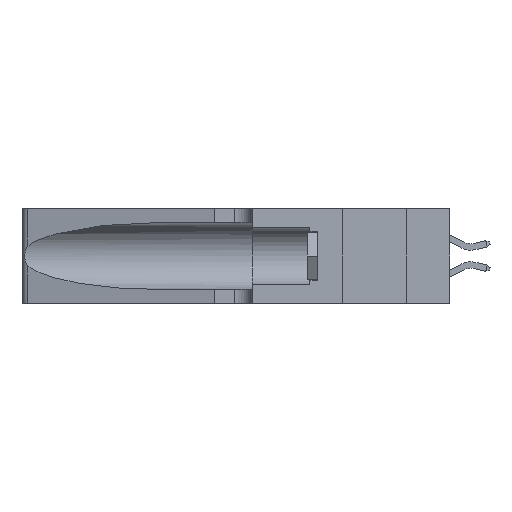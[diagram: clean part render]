
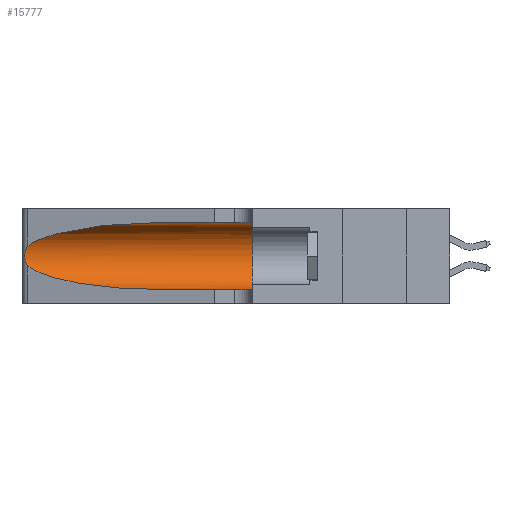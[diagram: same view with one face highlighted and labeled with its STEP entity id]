
A CAD part, left-side view. The second image highlights one B-rep face of the part: STEP entity #15777.
In plain terms, the highlighted cylindrical face has radius 3.308 mm (diameter 6.617 mm), a partial arc.
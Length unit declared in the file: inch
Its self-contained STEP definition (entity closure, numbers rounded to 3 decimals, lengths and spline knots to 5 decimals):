
#807 = DIRECTION ( 'NONE',  ( 0., -1., 0. ) ) ;
#808 = AXIS2_PLACEMENT_3D ( 'NONE', #12505, #12678, #12764 ) ;
#862 = CARTESIAN_POINT ( 'NONE',  ( 0.18966, 0.96281, 0.05475 ) ) ;
#995 = EDGE_CURVE ( 'NONE', #19436, #9835, #7386, .T. ) ;
#1857 = CARTESIAN_POINT ( 'NONE',  ( 0.25854, 1.2359, 0.20912 ) ) ;
#1946 = CARTESIAN_POINT ( 'NONE',  ( 0.26075, 1.23896, 0.178 ) ) ;
#2101 = CARTESIAN_POINT ( 'NONE',  ( 0.26017, 1.23833, 0.17102 ) ) ;
#2429 = VECTOR ( 'NONE', #807, 39.37008 ) ;
#4340 = CARTESIAN_POINT ( 'NONE',  ( 0.1305, 0.72297, 0.05475 ) ) ;
#4349 = CARTESIAN_POINT ( 'NONE',  ( 0.1305, 0.35, 0.31525 ) ) ;
#5874 = CARTESIAN_POINT ( 'NONE',  ( 0.1305, 1.61858, 0.31525 ) ) ;
#6465 = EDGE_LOOP ( 'NONE', ( #8279, #24829, #11909, #16820, #25106, #7461 ) ) ;
#6874 = EDGE_CURVE ( 'NONE', #16310, #11037, #12631, .T. ) ;
#6916 =( BOUNDED_CURVE ( )  B_SPLINE_CURVE ( 3, ( #19974, #18110, #862, #18564 ),
 .UNSPECIFIED., .F., .T. ) 
 B_SPLINE_CURVE_WITH_KNOTS ( ( 4, 4 ),
 ( 3.44316, 4.71239 ),
 .UNSPECIFIED. ) 
 CURVE ( )  GEOMETRIC_REPRESENTATION_ITEM ( )  RATIONAL_B_SPLINE_CURVE ( ( 1., 0.87, 0.87, 1. ) ) 
 REPRESENTATION_ITEM ( '' )  );
#7386 = B_SPLINE_CURVE_WITH_KNOTS ( 'NONE', 3,
 ( #21714, #17870, #23707, #9993, #1857, #23624, #19993, #1946, #2101, #13982, #15690, #25715, #15786, #7904 ),
 .UNSPECIFIED., .F., .F.,
 ( 4, 2, 2, 2, 2, 2, 4 ),
 ( 0., 0.00027, 0.00053, 0.00107, 0.0016, 0.00187, 0.00214 ),
 .UNSPECIFIED. ) ;
#7461 = ORIENTED_EDGE ( 'NONE', *, *, #15427, .F. ) ;
#7904 = CARTESIAN_POINT ( 'NONE',  ( 0.25487, 1.22718, 0.14631 ) ) ;
#8279 = ORIENTED_EDGE ( 'NONE', *, *, #11828, .T. ) ;
#8704 = DIRECTION ( 'NONE',  ( 0., 0., 1. ) ) ;
#9835 = VERTEX_POINT ( 'NONE', #12852 ) ;
#9993 = CARTESIAN_POINT ( 'NONE',  ( 0.25787, 1.23484, 0.2124 ) ) ;
#10057 = CARTESIAN_POINT ( 'NONE',  ( 0.25487, 1.22718, 0.22369 ) ) ;
#10873 =( BOUNDED_CURVE ( )  B_SPLINE_CURVE ( 3, ( #22787, #15052, #18729, #24969 ),
 .UNSPECIFIED., .F., .F. ) 
 B_SPLINE_CURVE_WITH_KNOTS ( ( 4, 4 ),
 ( 1.5708, 2.84003 ),
 .UNSPECIFIED. ) 
 CURVE ( )  GEOMETRIC_REPRESENTATION_ITEM ( )  RATIONAL_B_SPLINE_CURVE ( ( 1., 0.87, 0.87, 1. ) ) 
 REPRESENTATION_ITEM ( '' )  );
#11037 = VERTEX_POINT ( 'NONE', #16438 ) ;
#11586 = CYLINDRICAL_SURFACE ( 'NONE', #808, 0.13025 ) ;
#11828 = EDGE_CURVE ( 'NONE', #23755, #19436, #10873, .T. ) ;
#11909 = ORIENTED_EDGE ( 'NONE', *, *, #12552, .T. ) ;
#12505 = CARTESIAN_POINT ( 'NONE',  ( 0.1305, 1.61858, 0.185 ) ) ;
#12552 = EDGE_CURVE ( 'NONE', #9835, #16310, #6916, .T. ) ;
#12631 = LINE ( 'NONE', #16578, #2429 ) ;
#12678 = DIRECTION ( 'NONE',  ( 0., -1., 0. ) ) ;
#12764 = DIRECTION ( 'NONE',  ( 0., 0., -1. ) ) ;
#12852 = CARTESIAN_POINT ( 'NONE',  ( 0.25487, 1.22718, 0.14631 ) ) ;
#13520 = DIRECTION ( 'NONE',  ( 0., -1., 0. ) ) ;
#13982 = CARTESIAN_POINT ( 'NONE',  ( 0.25856, 1.23593, 0.16098 ) ) ;
#15052 = CARTESIAN_POINT ( 'NONE',  ( 0.18966, 0.96281, 0.31525 ) ) ;
#15427 = EDGE_CURVE ( 'NONE', #23755, #18239, #17205, .T. ) ;
#15690 = CARTESIAN_POINT ( 'NONE',  ( 0.25789, 1.23486, 0.15765 ) ) ;
#15777 = ADVANCED_FACE ( 'NONE', ( #24671 ), #11586, .F. ) ;
#15786 = CARTESIAN_POINT ( 'NONE',  ( 0.25555, 1.22993, 0.14849 ) ) ;
#16310 = VERTEX_POINT ( 'NONE', #4340 ) ;
#16438 = CARTESIAN_POINT ( 'NONE',  ( 0.1305, 0.35, 0.05475 ) ) ;
#16578 = CARTESIAN_POINT ( 'NONE',  ( 0.1305, 1.61858, 0.05475 ) ) ;
#16820 = ORIENTED_EDGE ( 'NONE', *, *, #6874, .T. ) ;
#17205 = LINE ( 'NONE', #5874, #19716 ) ;
#17869 = EDGE_CURVE ( 'NONE', #18239, #11037, #23369, .T. ) ;
#17870 = CARTESIAN_POINT ( 'NONE',  ( 0.25555, 1.22994, 0.2215 ) ) ;
#18110 = CARTESIAN_POINT ( 'NONE',  ( 0.2373, 1.15595, 0.08982 ) ) ;
#18239 = VERTEX_POINT ( 'NONE', #4349 ) ;
#18487 = CARTESIAN_POINT ( 'NONE',  ( 0.1305, 0.35, 0.185 ) ) ;
#18564 = CARTESIAN_POINT ( 'NONE',  ( 0.1305, 0.72297, 0.05475 ) ) ;
#18679 = DIRECTION ( 'NONE',  ( 0., 1., 0. ) ) ;
#18729 = CARTESIAN_POINT ( 'NONE',  ( 0.2373, 1.15595, 0.28018 ) ) ;
#19436 = VERTEX_POINT ( 'NONE', #10057 ) ;
#19716 = VECTOR ( 'NONE', #13520, 39.37008 ) ;
#19974 = CARTESIAN_POINT ( 'NONE',  ( 0.25487, 1.22718, 0.14631 ) ) ;
#19993 = CARTESIAN_POINT ( 'NONE',  ( 0.26075, 1.23896, 0.19203 ) ) ;
#20678 = CARTESIAN_POINT ( 'NONE',  ( 0.1305, 0.72297, 0.31525 ) ) ;
#21714 = CARTESIAN_POINT ( 'NONE',  ( 0.25487, 1.22718, 0.22369 ) ) ;
#22787 = CARTESIAN_POINT ( 'NONE',  ( 0.1305, 0.72297, 0.31525 ) ) ;
#23111 = AXIS2_PLACEMENT_3D ( 'NONE', #18487, #18679, #8704 ) ;
#23369 = CIRCLE ( 'NONE', #23111, 0.13025 ) ;
#23624 = CARTESIAN_POINT ( 'NONE',  ( 0.26018, 1.23835, 0.19895 ) ) ;
#23707 = CARTESIAN_POINT ( 'NONE',  ( 0.25639, 1.23184, 0.21858 ) ) ;
#23755 = VERTEX_POINT ( 'NONE', #20678 ) ;
#24671 = FACE_OUTER_BOUND ( 'NONE', #6465, .T. ) ;
#24829 = ORIENTED_EDGE ( 'NONE', *, *, #995, .T. ) ;
#24969 = CARTESIAN_POINT ( 'NONE',  ( 0.25487, 1.22718, 0.22369 ) ) ;
#25106 = ORIENTED_EDGE ( 'NONE', *, *, #17869, .F. ) ;
#25715 = CARTESIAN_POINT ( 'NONE',  ( 0.25639, 1.23186, 0.15144 ) ) ;
